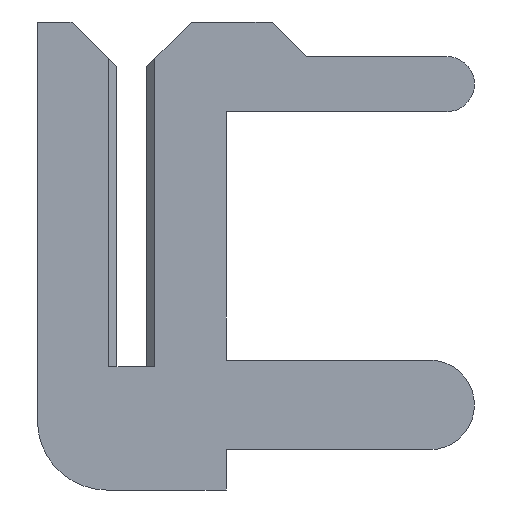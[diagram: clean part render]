
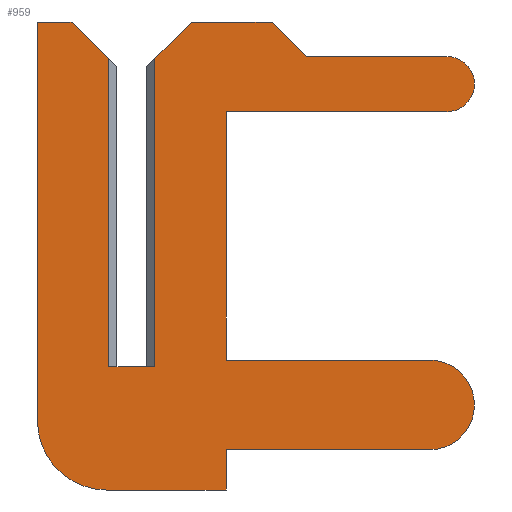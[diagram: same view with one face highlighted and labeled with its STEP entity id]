
A CAD part, left-side view. The second image highlights one B-rep face of the part: STEP entity #959.
In plain terms, the highlighted planar face has unit normal (-1, 0, 0).
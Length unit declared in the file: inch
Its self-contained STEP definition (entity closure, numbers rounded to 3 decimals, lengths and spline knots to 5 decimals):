
#1 = CARTESIAN_POINT ( 'NONE',  ( -0.01, -0.041, -0.036 ) ) ;
#8 = DIRECTION ( 'NONE',  ( 0., -0.707, -0.707 ) ) ;
#16 = LINE ( 'NONE', #477, #987 ) ;
#21 = CARTESIAN_POINT ( 'NONE',  ( -0.01, -0.041, 0.003 ) ) ;
#32 = VERTEX_POINT ( 'NONE', #1396 ) ;
#50 = AXIS2_PLACEMENT_3D ( 'NONE', #674, #1016, #910 ) ;
#63 = CARTESIAN_POINT ( 'NONE',  ( -0.01, 0.011, -0.0235 ) ) ;
#76 = EDGE_CURVE ( 'NONE', #650, #32, #473, .T. ) ;
#109 = LINE ( 'NONE', #727, #836 ) ;
#113 = DIRECTION ( 'NONE',  ( 0., 1., 0. ) ) ;
#118 = DIRECTION ( 'NONE',  ( 0., -0.707, -0.707 ) ) ;
#125 = CARTESIAN_POINT ( 'NONE',  ( -0.01, -0.1295, 0.003 ) ) ;
#133 = CARTESIAN_POINT ( 'NONE',  ( -0.01, -0.076, 0.135 ) ) ;
#138 = CARTESIAN_POINT ( 'NONE',  ( -0.01, 0.026, 0.15 ) ) ;
#171 = ORIENTED_EDGE ( 'NONE', *, *, #1288, .F. ) ;
#182 = LINE ( 'NONE', #913, #1162 ) ;
#185 = PLANE ( 'NONE',  #1028 ) ;
#191 = ORIENTED_EDGE ( 'NONE', *, *, #248, .F. ) ;
#196 = CARTESIAN_POINT ( 'NONE',  ( -0.01, -0.061, 0.15 ) ) ;
#220 = EDGE_CURVE ( 'NONE', #1187, #757, #182, .T. ) ;
#226 = AXIS2_PLACEMENT_3D ( 'NONE', #323, #1277, #1091 ) ;
#233 = CARTESIAN_POINT ( 'NONE',  ( -0.01, 0.041, -0.0235 ) ) ;
#234 = VECTOR ( 'NONE', #8, 39.37008 ) ;
#248 = EDGE_CURVE ( 'NONE', #388, #1094, #16, .T. ) ;
#254 = DIRECTION ( 'NONE',  ( 0., 0., -1. ) ) ;
#268 = VERTEX_POINT ( 'NONE', #21 ) ;
#272 = CARTESIAN_POINT ( 'NONE',  ( -0.01, -0.041, 0.111 ) ) ;
#279 = FACE_OUTER_BOUND ( 'NONE', #541, .T. ) ;
#283 = CARTESIAN_POINT ( 'NONE',  ( -0.01, -0.076, 0.135 ) ) ;
#293 = CARTESIAN_POINT ( 'NONE',  ( -0.01, 0.011, -0.0235 ) ) ;
#298 = EDGE_CURVE ( 'NONE', #32, #844, #643, .T. ) ;
#301 = CARTESIAN_POINT ( 'NONE',  ( -0.01, -0.1295, 0.003 ) ) ;
#303 = DIRECTION ( 'NONE',  ( -1., 0., 0. ) ) ;
#304 = LINE ( 'NONE', #861, #922 ) ;
#312 = VERTEX_POINT ( 'NONE', #1002 ) ;
#318 = VECTOR ( 'NONE', #1343, 39.37008 ) ;
#323 = CARTESIAN_POINT ( 'NONE',  ( -0.01, -0.1295, -0.0165 ) ) ;
#332 = ORIENTED_EDGE ( 'NONE', *, *, #627, .F. ) ;
#337 = DIRECTION ( 'NONE',  ( 0., -0.707, 0.707 ) ) ;
#349 = LINE ( 'NONE', #489, #318 ) ;
#356 = ORIENTED_EDGE ( 'NONE', *, *, #1217, .T. ) ;
#369 = LINE ( 'NONE', #272, #1376 ) ;
#371 = EDGE_CURVE ( 'NONE', #1222, #701, #580, .T. ) ;
#372 = DIRECTION ( 'NONE',  ( 0., -1., 0. ) ) ;
#388 = VERTEX_POINT ( 'NONE', #583 ) ;
#401 = DIRECTION ( 'NONE',  ( 1., 0., 0. ) ) ;
#404 = ORIENTED_EDGE ( 'NONE', *, *, #700, .F. ) ;
#419 = ORIENTED_EDGE ( 'NONE', *, *, #371, .F. ) ;
#425 = CIRCLE ( 'NONE', #750, 0.03 ) ;
#431 = DIRECTION ( 'NONE',  ( 0., 0., 1. ) ) ;
#473 = LINE ( 'NONE', #652, #1269 ) ;
#477 = CARTESIAN_POINT ( 'NONE',  ( -0.01, 0.0065, 0. ) ) ;
#486 = EDGE_CURVE ( 'NONE', #811, #268, #967, .T. ) ;
#489 = CARTESIAN_POINT ( 'NONE',  ( -0.01, 0.011, -0.0535 ) ) ;
#522 = VERTEX_POINT ( 'NONE', #283 ) ;
#531 = CARTESIAN_POINT ( 'NONE',  ( -0.01, 0.011, -0.0535 ) ) ;
#532 = VECTOR ( 'NONE', #118, 39.37008 ) ;
#536 = CIRCLE ( 'NONE', #226, 0.0195 ) ;
#541 = EDGE_LOOP ( 'NONE', ( #1235, #830, #191, #356, #332, #893, #573, #978, #657, #699, #1386, #171, #404, #1054, #592, #419, #1073, #1249, #820 ) ) ;
#543 = VERTEX_POINT ( 'NONE', #1357 ) ;
#573 = ORIENTED_EDGE ( 'NONE', *, *, #76, .F. ) ;
#580 = CIRCLE ( 'NONE', #50, 0.012 ) ;
#582 = EDGE_CURVE ( 'NONE', #701, #811, #369, .T. ) ;
#583 = CARTESIAN_POINT ( 'NONE',  ( -0.01, 0.01, 0. ) ) ;
#592 = ORIENTED_EDGE ( 'NONE', *, *, #582, .F. ) ;
#627 = EDGE_CURVE ( 'NONE', #844, #543, #935, .T. ) ;
#642 = VECTOR ( 'NONE', #779, 39.37008 ) ;
#643 = LINE ( 'NONE', #687, #1293 ) ;
#650 = VERTEX_POINT ( 'NONE', #233 ) ;
#652 = CARTESIAN_POINT ( 'NONE',  ( -0.01, 0.041, 0.15 ) ) ;
#657 = ORIENTED_EDGE ( 'NONE', *, *, #923, .F. ) ;
#661 = VERTEX_POINT ( 'NONE', #906 ) ;
#664 = CARTESIAN_POINT ( 'NONE',  ( -0.01, -0.041, -0.0535 ) ) ;
#667 = DIRECTION ( 'NONE',  ( 0., 1., 0. ) ) ;
#669 = EDGE_CURVE ( 'NONE', #739, #1187, #1192, .T. ) ;
#670 = VECTOR ( 'NONE', #667, 39.37008 ) ;
#674 = CARTESIAN_POINT ( 'NONE',  ( -0.01, -0.137, 0.123 ) ) ;
#687 = CARTESIAN_POINT ( 'NONE',  ( -0.01, 0.026, 0.15 ) ) ;
#694 = DIRECTION ( 'NONE',  ( 0., -1., 0. ) ) ;
#699 = ORIENTED_EDGE ( 'NONE', *, *, #220, .F. ) ;
#700 = EDGE_CURVE ( 'NONE', #268, #897, #855, .T. ) ;
#701 = VERTEX_POINT ( 'NONE', #794 ) ;
#711 = DIRECTION ( 'NONE',  ( 0., -1., 0. ) ) ;
#718 = EDGE_CURVE ( 'NONE', #1236, #522, #831, .T. ) ;
#727 = CARTESIAN_POINT ( 'NONE',  ( -0.01, -0.026, 0.15 ) ) ;
#733 = VECTOR ( 'NONE', #337, 39.37008 ) ;
#739 = VERTEX_POINT ( 'NONE', #1000 ) ;
#745 = DIRECTION ( 'NONE',  ( 0., -1., 0. ) ) ;
#750 = AXIS2_PLACEMENT_3D ( 'NONE', #63, #401, #1158 ) ;
#757 = VERTEX_POINT ( 'NONE', #664 ) ;
#766 = DIRECTION ( 'NONE',  ( 0., 0., 1. ) ) ;
#779 = DIRECTION ( 'NONE',  ( 0., -1., 0. ) ) ;
#792 = CARTESIAN_POINT ( 'NONE',  ( -0.01, -0.041, 0.003 ) ) ;
#794 = CARTESIAN_POINT ( 'NONE',  ( -0.01, -0.137, 0.111 ) ) ;
#799 = LINE ( 'NONE', #971, #733 ) ;
#811 = VERTEX_POINT ( 'NONE', #1111 ) ;
#816 = LINE ( 'NONE', #1047, #1027 ) ;
#820 = ORIENTED_EDGE ( 'NONE', *, *, #1174, .F. ) ;
#824 = DIRECTION ( 'NONE',  ( 0., 0., 1. ) ) ;
#830 = ORIENTED_EDGE ( 'NONE', *, *, #1280, .T. ) ;
#831 = LINE ( 'NONE', #133, #234 ) ;
#836 = VECTOR ( 'NONE', #745, 39.37008 ) ;
#844 = VERTEX_POINT ( 'NONE', #138 ) ;
#855 = LINE ( 'NONE', #125, #642 ) ;
#861 = CARTESIAN_POINT ( 'NONE',  ( -0.01, 0.01, -0.0235 ) ) ;
#893 = ORIENTED_EDGE ( 'NONE', *, *, #298, .F. ) ;
#897 = VERTEX_POINT ( 'NONE', #301 ) ;
#906 = CARTESIAN_POINT ( 'NONE',  ( -0.01, -0.026, 0.15 ) ) ;
#910 = DIRECTION ( 'NONE',  ( 0., 0., 1. ) ) ;
#913 = CARTESIAN_POINT ( 'NONE',  ( -0.01, -0.041, -0.0535 ) ) ;
#922 = VECTOR ( 'NONE', #431, 39.37008 ) ;
#923 = EDGE_CURVE ( 'NONE', #757, #1138, #349, .T. ) ;
#935 = LINE ( 'NONE', #1123, #532 ) ;
#953 = CARTESIAN_POINT ( 'NONE',  ( -0.01, -0.137, 0.135 ) ) ;
#959 = ADVANCED_FACE ( 'NONE', ( #279 ), #185, .T. ) ;
#967 = LINE ( 'NONE', #792, #1270 ) ;
#971 = CARTESIAN_POINT ( 'NONE',  ( -0.01, -0.0065, 0.1305 ) ) ;
#978 = ORIENTED_EDGE ( 'NONE', *, *, #1056, .F. ) ;
#987 = VECTOR ( 'NONE', #372, 39.37008 ) ;
#1000 = CARTESIAN_POINT ( 'NONE',  ( -0.01, -0.1295, -0.036 ) ) ;
#1002 = CARTESIAN_POINT ( 'NONE',  ( -0.01, -0.01, 0.134 ) ) ;
#1016 = DIRECTION ( 'NONE',  ( 1., 0., 0. ) ) ;
#1027 = VECTOR ( 'NONE', #711, 39.37008 ) ;
#1028 = AXIS2_PLACEMENT_3D ( 'NONE', #293, #303, #824 ) ;
#1047 = CARTESIAN_POINT ( 'NONE',  ( -0.01, -0.137, 0.135 ) ) ;
#1054 = ORIENTED_EDGE ( 'NONE', *, *, #486, .F. ) ;
#1056 = EDGE_CURVE ( 'NONE', #1138, #650, #425, .T. ) ;
#1072 = CARTESIAN_POINT ( 'NONE',  ( -0.01, -0.01, 0.15 ) ) ;
#1073 = ORIENTED_EDGE ( 'NONE', *, *, #1389, .F. ) ;
#1091 = DIRECTION ( 'NONE',  ( 0., 0., 1. ) ) ;
#1094 = VERTEX_POINT ( 'NONE', #1274 ) ;
#1111 = CARTESIAN_POINT ( 'NONE',  ( -0.01, -0.041, 0.111 ) ) ;
#1123 = CARTESIAN_POINT ( 'NONE',  ( -0.01, 0.0065, 0.1305 ) ) ;
#1132 = DIRECTION ( 'NONE',  ( 0., 0., -1. ) ) ;
#1138 = VERTEX_POINT ( 'NONE', #531 ) ;
#1158 = DIRECTION ( 'NONE',  ( 0., 0., 1. ) ) ;
#1162 = VECTOR ( 'NONE', #254, 39.37008 ) ;
#1174 = EDGE_CURVE ( 'NONE', #661, #1236, #109, .T. ) ;
#1177 = DIRECTION ( 'NONE',  ( 0., 0., -1. ) ) ;
#1182 = VECTOR ( 'NONE', #1177, 39.37008 ) ;
#1187 = VERTEX_POINT ( 'NONE', #1412 ) ;
#1192 = LINE ( 'NONE', #1, #670 ) ;
#1217 = EDGE_CURVE ( 'NONE', #388, #543, #304, .T. ) ;
#1222 = VERTEX_POINT ( 'NONE', #953 ) ;
#1235 = ORIENTED_EDGE ( 'NONE', *, *, #1271, .F. ) ;
#1236 = VERTEX_POINT ( 'NONE', #196 ) ;
#1249 = ORIENTED_EDGE ( 'NONE', *, *, #718, .F. ) ;
#1269 = VECTOR ( 'NONE', #766, 39.37008 ) ;
#1270 = VECTOR ( 'NONE', #1132, 39.37008 ) ;
#1271 = EDGE_CURVE ( 'NONE', #312, #661, #799, .T. ) ;
#1274 = CARTESIAN_POINT ( 'NONE',  ( -0.01, -0.01, 0. ) ) ;
#1277 = DIRECTION ( 'NONE',  ( 1., 0., 0. ) ) ;
#1280 = EDGE_CURVE ( 'NONE', #312, #1094, #1352, .T. ) ;
#1288 = EDGE_CURVE ( 'NONE', #897, #739, #536, .T. ) ;
#1293 = VECTOR ( 'NONE', #694, 39.37008 ) ;
#1343 = DIRECTION ( 'NONE',  ( 0., 1., 0. ) ) ;
#1352 = LINE ( 'NONE', #1072, #1182 ) ;
#1357 = CARTESIAN_POINT ( 'NONE',  ( -0.01, 0.01, 0.134 ) ) ;
#1376 = VECTOR ( 'NONE', #113, 39.37008 ) ;
#1386 = ORIENTED_EDGE ( 'NONE', *, *, #669, .F. ) ;
#1389 = EDGE_CURVE ( 'NONE', #522, #1222, #816, .T. ) ;
#1396 = CARTESIAN_POINT ( 'NONE',  ( -0.01, 0.041, 0.15 ) ) ;
#1412 = CARTESIAN_POINT ( 'NONE',  ( -0.01, -0.041, -0.036 ) ) ;
